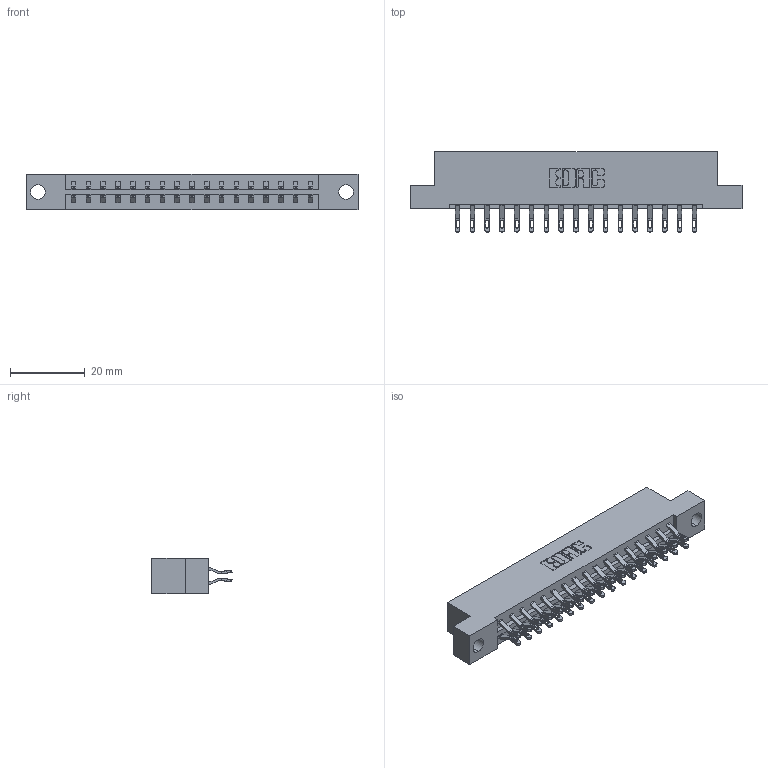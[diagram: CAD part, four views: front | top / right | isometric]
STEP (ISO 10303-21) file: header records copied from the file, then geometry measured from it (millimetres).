
FILE_DESCRIPTION (( 'STEP AP203' ), '1' );
FILE_NAME ('833-034-555-204.STEP', '2020-06-02T23:06:46', ( '' ), ( '' ), 'SwSTEP 2.0', 'SolidWorks 2020', '' );
FILE_SCHEMA (( 'CONFIG_CONTROL_DESIGN' ));
Length unit declared in the file: inch
Products named in the file (3): 833 Part_Flush - .156 Dia - TH; 833-034-555-204; 345-292-001_555 Tail
Assembly tree (35 placements, depth 2):
  833-034-555-204
    833 Part_Flush - .156 Dia - TH
    345-292-001_555 Tail  x34
Bounding box: 88.9 x 21.47 x 9.4 mm (x, y, z)
Volume: 8853.2 mm3; surface area: 10366.2 mm2
Topology: 35 solids, 35 shells, 2086 faces, 6533 edges, 4354 vertices
Faces by surface type: plane 1226, cylinder 860
Entity records: 14499 total; most frequent: CARTESIAN_POINT 2468, ORIENTED_EDGE 2374, DIRECTION 2123, EDGE_CURVE 1187, VECTOR 1039, LINE 1039, VERTEX_POINT 790, AXIS2_PLACEMENT_3D 542
